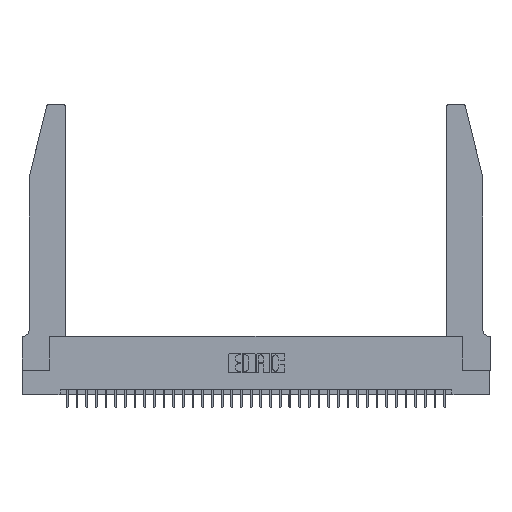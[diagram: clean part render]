
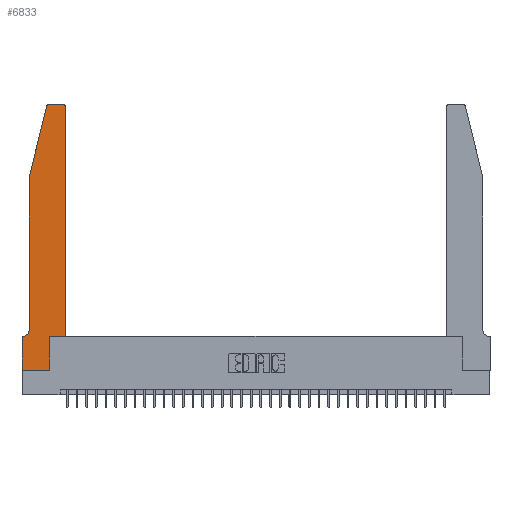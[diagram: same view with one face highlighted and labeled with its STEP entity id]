
A CAD part, top view. The second image highlights one B-rep face of the part: STEP entity #6833.
In plain terms, the highlighted planar face has unit normal (0, 0, 1).
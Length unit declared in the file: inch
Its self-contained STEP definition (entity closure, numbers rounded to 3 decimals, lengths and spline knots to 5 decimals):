
#236 = DIRECTION ( 'NONE',  ( 0., -1., 0. ) ) ;
#470 = CIRCLE ( 'NONE', #5203, 0.03 ) ;
#1010 = DIRECTION ( 'NONE',  ( 0., 0., -1. ) ) ;
#2219 = LINE ( 'NONE', #33448, #30089 ) ;
#2582 = ORIENTED_EDGE ( 'NONE', *, *, #34342, .T. ) ;
#3401 = VECTOR ( 'NONE', #23816, 39.37008 ) ;
#3418 = LINE ( 'NONE', #11931, #31393 ) ;
#3645 = DIRECTION ( 'NONE',  ( 1., 0., 0. ) ) ;
#3821 = CARTESIAN_POINT ( 'NONE',  ( 0.4205, 2.72, 0.37 ) ) ;
#4702 = DIRECTION ( 'NONE',  ( -1., 0., 0. ) ) ;
#5203 = AXIS2_PLACEMENT_3D ( 'NONE', #3821, #17717, #3645 ) ;
#5663 = EDGE_CURVE ( 'NONE', #18406, #10931, #470, .T. ) ;
#5770 = DIRECTION ( 'NONE',  ( -0.239, -0.971, 0. ) ) ;
#6833 = ADVANCED_FACE ( 'NONE', ( #17813 ), #23150, .T. ) ;
#6863 = ORIENTED_EDGE ( 'NONE', *, *, #18948, .T. ) ;
#7533 = DIRECTION ( 'NONE',  ( 0., 0., 1. ) ) ;
#7860 = VERTEX_POINT ( 'NONE', #19772 ) ;
#7862 = ORIENTED_EDGE ( 'NONE', *, *, #25204, .T. ) ;
#8008 = LINE ( 'NONE', #19300, #28072 ) ;
#8079 = ORIENTED_EDGE ( 'NONE', *, *, #19387, .T. ) ;
#8101 = CARTESIAN_POINT ( 'NONE',  ( 0., 0.35, 0.37 ) ) ;
#8447 = VERTEX_POINT ( 'NONE', #20103 ) ;
#8572 = DIRECTION ( 'NONE',  ( -1., 0., 0. ) ) ;
#8650 = ORIENTED_EDGE ( 'NONE', *, *, #18219, .T. ) ;
#8913 = DIRECTION ( 'NONE',  ( 0., 0., 1. ) ) ;
#9420 = CARTESIAN_POINT ( 'NONE',  ( 0.0755, 0.35, 0.37 ) ) ;
#9476 = EDGE_CURVE ( 'NONE', #26517, #31369, #17544, .T. ) ;
#10160 = VECTOR ( 'NONE', #18487, 39.37008 ) ;
#10931 = VERTEX_POINT ( 'NONE', #12931 ) ;
#10964 = VECTOR ( 'NONE', #8572, 39.37008 ) ;
#11278 = VECTOR ( 'NONE', #236, 39.37008 ) ;
#11569 = VERTEX_POINT ( 'NONE', #27424 ) ;
#11805 = CIRCLE ( 'NONE', #35421, 0.07 ) ;
#11931 = CARTESIAN_POINT ( 'NONE',  ( 0.4505, 0.35, 0.37 ) ) ;
#12037 = DIRECTION ( 'NONE',  ( 1., 0., 0. ) ) ;
#12743 = LINE ( 'NONE', #9420, #3401 ) ;
#12856 = ORIENTED_EDGE ( 'NONE', *, *, #35028, .T. ) ;
#12931 = CARTESIAN_POINT ( 'NONE',  ( 0.4205, 2.75, 0.37 ) ) ;
#13668 = EDGE_CURVE ( 'NONE', #17130, #18406, #3418, .T. ) ;
#13977 = CARTESIAN_POINT ( 'NONE',  ( 0.2605, 2.75, 0.37 ) ) ;
#14226 = EDGE_CURVE ( 'NONE', #23656, #17130, #32373, .T. ) ;
#14711 = CARTESIAN_POINT ( 'NONE',  ( 0., 0., 0.37 ) ) ;
#15064 = CARTESIAN_POINT ( 'NONE',  ( 0., 0.35, 0.37 ) ) ;
#15570 = DIRECTION ( 'NONE',  ( 0., 1., 0. ) ) ;
#16101 = CARTESIAN_POINT ( 'NONE',  ( 0.284, 2.75, 0.37 ) ) ;
#16163 = VERTEX_POINT ( 'NONE', #25712 ) ;
#16326 = AXIS2_PLACEMENT_3D ( 'NONE', #15064, #8913, #12037 ) ;
#17130 = VERTEX_POINT ( 'NONE', #22940 ) ;
#17544 = CIRCLE ( 'NONE', #30474, 0.03 ) ;
#17717 = DIRECTION ( 'NONE',  ( 0., 0., 1. ) ) ;
#17813 = FACE_OUTER_BOUND ( 'NONE', #36500, .T. ) ;
#18219 = EDGE_CURVE ( 'NONE', #31369, #8447, #8008, .T. ) ;
#18406 = VERTEX_POINT ( 'NONE', #30159 ) ;
#18473 = LINE ( 'NONE', #29743, #32235 ) ;
#18487 = DIRECTION ( 'NONE',  ( 1., 0., 0. ) ) ;
#18678 = EDGE_CURVE ( 'NONE', #25257, #23656, #18473, .T. ) ;
#18827 = DIRECTION ( 'NONE',  ( 1., 0., 0. ) ) ;
#18844 = CARTESIAN_POINT ( 'NONE',  ( 0.2865, 0.35, 0.37 ) ) ;
#18948 = EDGE_CURVE ( 'NONE', #10931, #26517, #33896, .T. ) ;
#19300 = CARTESIAN_POINT ( 'NONE',  ( 0.0755, 2., 0.37 ) ) ;
#19387 = EDGE_CURVE ( 'NONE', #8447, #16163, #2219, .T. ) ;
#19772 = CARTESIAN_POINT ( 'NONE',  ( 0., 0., 0.37 ) ) ;
#20103 = CARTESIAN_POINT ( 'NONE',  ( 0.0755, 2., 0.37 ) ) ;
#21917 = VECTOR ( 'NONE', #23035, 39.37008 ) ;
#22732 = ORIENTED_EDGE ( 'NONE', *, *, #5663, .T. ) ;
#22896 = ORIENTED_EDGE ( 'NONE', *, *, #14226, .T. ) ;
#22940 = CARTESIAN_POINT ( 'NONE',  ( 0.4505, 0.35, 0.37 ) ) ;
#23035 = DIRECTION ( 'NONE',  ( 1., 0., 0. ) ) ;
#23150 = PLANE ( 'NONE',  #16326 ) ;
#23573 = ORIENTED_EDGE ( 'NONE', *, *, #9476, .T. ) ;
#23582 = LINE ( 'NONE', #26360, #21917 ) ;
#23656 = VERTEX_POINT ( 'NONE', #18844 ) ;
#23816 = DIRECTION ( 'NONE',  ( -1., 0., 0. ) ) ;
#24533 = CARTESIAN_POINT ( 'NONE',  ( 0.284, 2.72, 0.37 ) ) ;
#25204 = EDGE_CURVE ( 'NONE', #11569, #26705, #12743, .T. ) ;
#25257 = VERTEX_POINT ( 'NONE', #31775 ) ;
#25712 = CARTESIAN_POINT ( 'NONE',  ( 0.0755, 0.42, 0.37 ) ) ;
#26353 = CARTESIAN_POINT ( 'NONE',  ( 0.0055, 0.42, 0.37 ) ) ;
#26360 = CARTESIAN_POINT ( 'NONE',  ( 0., 0., 0.37 ) ) ;
#26385 = ORIENTED_EDGE ( 'NONE', *, *, #13668, .T. ) ;
#26517 = VERTEX_POINT ( 'NONE', #16101 ) ;
#26705 = VERTEX_POINT ( 'NONE', #8101 ) ;
#27424 = CARTESIAN_POINT ( 'NONE',  ( 0.0055, 0.35, 0.37 ) ) ;
#27522 = DIRECTION ( 'NONE',  ( 0., -1., 0. ) ) ;
#27936 = ORIENTED_EDGE ( 'NONE', *, *, #30875, .T. ) ;
#27996 = DIRECTION ( 'NONE',  ( 0., 1., 0. ) ) ;
#28072 = VECTOR ( 'NONE', #5770, 39.37008 ) ;
#29743 = CARTESIAN_POINT ( 'NONE',  ( 0.2865, 0.35, 0.37 ) ) ;
#30089 = VECTOR ( 'NONE', #27522, 39.37008 ) ;
#30136 = ORIENTED_EDGE ( 'NONE', *, *, #18678, .T. ) ;
#30159 = CARTESIAN_POINT ( 'NONE',  ( 0.4505, 2.72, 0.37 ) ) ;
#30474 = AXIS2_PLACEMENT_3D ( 'NONE', #24533, #7533, #18827 ) ;
#30875 = EDGE_CURVE ( 'NONE', #16163, #11569, #11805, .T. ) ;
#31369 = VERTEX_POINT ( 'NONE', #32402 ) ;
#31393 = VECTOR ( 'NONE', #27996, 39.37008 ) ;
#31775 = CARTESIAN_POINT ( 'NONE',  ( 0.2865, 0., 0.37 ) ) ;
#32032 = LINE ( 'NONE', #14711, #11278 ) ;
#32235 = VECTOR ( 'NONE', #15570, 39.37008 ) ;
#32373 = LINE ( 'NONE', #32566, #10160 ) ;
#32402 = CARTESIAN_POINT ( 'NONE',  ( 0.25487, 2.72718, 0.37 ) ) ;
#32566 = CARTESIAN_POINT ( 'NONE',  ( 0.4505, 0.35, 0.37 ) ) ;
#33448 = CARTESIAN_POINT ( 'NONE',  ( 0.0755, 2., 0.37 ) ) ;
#33896 = LINE ( 'NONE', #13977, #10964 ) ;
#34342 = EDGE_CURVE ( 'NONE', #26705, #7860, #32032, .T. ) ;
#35028 = EDGE_CURVE ( 'NONE', #7860, #25257, #23582, .T. ) ;
#35421 = AXIS2_PLACEMENT_3D ( 'NONE', #26353, #1010, #4702 ) ;
#36500 = EDGE_LOOP ( 'NONE', ( #6863, #23573, #8650, #8079, #27936, #7862, #2582, #12856, #30136, #22896, #26385, #22732 ) ) ;
